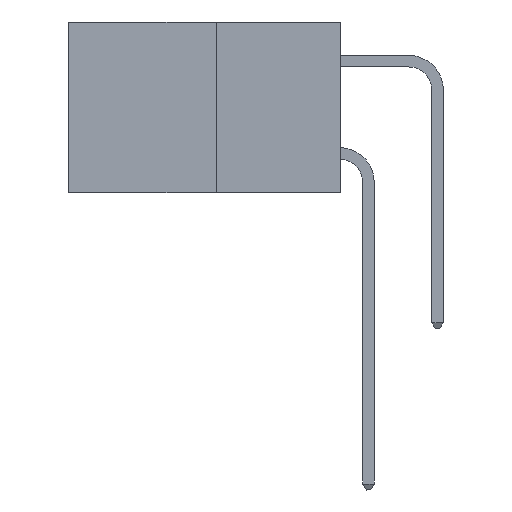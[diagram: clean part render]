
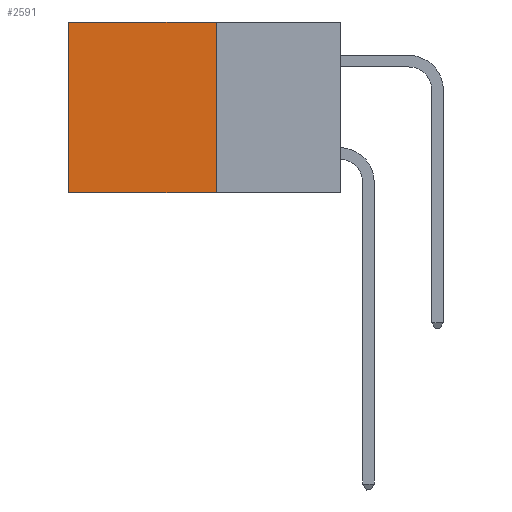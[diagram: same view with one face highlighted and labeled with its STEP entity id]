
A CAD part, left-side view. The second image highlights one B-rep face of the part: STEP entity #2591.
In plain terms, the highlighted planar face has unit normal (-1, 0, 0).
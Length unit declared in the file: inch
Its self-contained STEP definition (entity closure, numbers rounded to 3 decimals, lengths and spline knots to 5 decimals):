
#543 = EDGE_CURVE ( 'NONE', #6334, #571, #13472, .T. ) ;
#571 = VERTEX_POINT ( 'NONE', #7022 ) ;
#655 = VECTOR ( 'NONE', #5734, 39.37008 ) ;
#823 = DIRECTION ( 'NONE',  ( 0., 0., -1. ) ) ;
#2591 = ADVANCED_FACE ( 'NONE', ( #10226 ), #4337, .F. ) ;
#3018 = LINE ( 'NONE', #10718, #5861 ) ;
#3276 = DIRECTION ( 'NONE',  ( 0., 0., -1. ) ) ;
#4246 = DIRECTION ( 'NONE',  ( 1., 0., 0. ) ) ;
#4337 = PLANE ( 'NONE',  #11591 ) ;
#4430 = DIRECTION ( 'NONE',  ( 0., 0., -1. ) ) ;
#4532 = CARTESIAN_POINT ( 'NONE',  ( 0.277, 0.27, 0. ) ) ;
#4562 = ORIENTED_EDGE ( 'NONE', *, *, #543, .T. ) ;
#5734 = DIRECTION ( 'NONE',  ( 0., 1., 0. ) ) ;
#5861 = VECTOR ( 'NONE', #3276, 39.37008 ) ;
#6334 = VERTEX_POINT ( 'NONE', #13558 ) ;
#6544 = LINE ( 'NONE', #15452, #12758 ) ;
#7022 = CARTESIAN_POINT ( 'NONE',  ( 0.277, 0.59, 0. ) ) ;
#7173 = CARTESIAN_POINT ( 'NONE',  ( 0.277, 0.59, -0.37 ) ) ;
#7755 = LINE ( 'NONE', #9399, #11086 ) ;
#9234 = EDGE_CURVE ( 'NONE', #6334, #13444, #3018, .T. ) ;
#9399 = CARTESIAN_POINT ( 'NONE',  ( 0.277, 0.27, -0.37 ) ) ;
#10207 = CARTESIAN_POINT ( 'NONE',  ( 0.277, 0.27, -0.37 ) ) ;
#10226 = FACE_OUTER_BOUND ( 'NONE', #14105, .T. ) ;
#10294 = CARTESIAN_POINT ( 'NONE',  ( 0.277, 0.27, -0.37 ) ) ;
#10672 = VERTEX_POINT ( 'NONE', #7173 ) ;
#10718 = CARTESIAN_POINT ( 'NONE',  ( 0.277, 0.27, -0.37 ) ) ;
#11086 = VECTOR ( 'NONE', #15238, 39.37008 ) ;
#11591 = AXIS2_PLACEMENT_3D ( 'NONE', #10207, #4246, #4430 ) ;
#11866 = EDGE_CURVE ( 'NONE', #571, #10672, #6544, .T. ) ;
#12758 = VECTOR ( 'NONE', #823, 39.37008 ) ;
#13444 = VERTEX_POINT ( 'NONE', #10294 ) ;
#13472 = LINE ( 'NONE', #4532, #655 ) ;
#13558 = CARTESIAN_POINT ( 'NONE',  ( 0.277, 0.27, 0. ) ) ;
#13673 = ORIENTED_EDGE ( 'NONE', *, *, #11866, .T. ) ;
#14105 = EDGE_LOOP ( 'NONE', ( #13673, #15157, #15160, #4562 ) ) ;
#14576 = EDGE_CURVE ( 'NONE', #13444, #10672, #7755, .T. ) ;
#15157 = ORIENTED_EDGE ( 'NONE', *, *, #14576, .F. ) ;
#15160 = ORIENTED_EDGE ( 'NONE', *, *, #9234, .F. ) ;
#15238 = DIRECTION ( 'NONE',  ( 0., 1., 0. ) ) ;
#15452 = CARTESIAN_POINT ( 'NONE',  ( 0.277, 0.59, -0.37 ) ) ;
